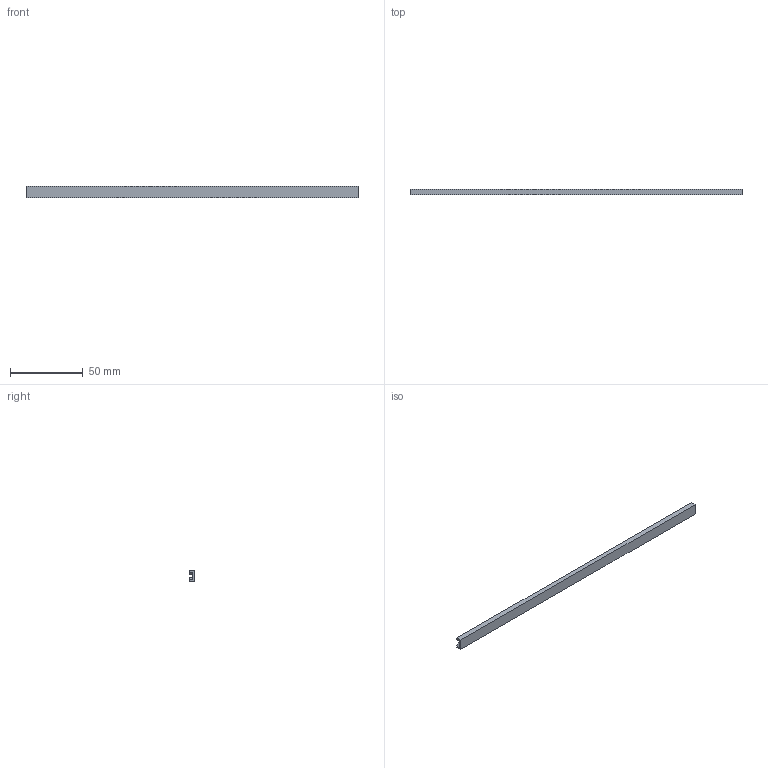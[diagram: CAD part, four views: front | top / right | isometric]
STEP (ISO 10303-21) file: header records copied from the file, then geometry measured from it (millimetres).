
FILE_DESCRIPTION (( 'STEP AP214' ), '1' );
FILE_NAME ('616-220-310.STEP', '2020-08-20T18:13:41', ( '' ), ( '' ), 'SwSTEP 2.0', 'SolidWorks 2020', '' );
FILE_SCHEMA (( 'AUTOMOTIVE_DESIGN' ));
Length unit declared in the file: inch
Products named in the file (1): 616-220-310
Bounding box: 228.6 x 3.71 x 7.92 mm (x, y, z)
Volume: 5534.2 mm3; surface area: 6360.8 mm2
Topology: 1 solids, 1 shells, 262 faces, 687 edges, 458 vertices
Faces by surface type: plane 168, bspline 94
Entity records: 13655 total; most frequent: CARTESIAN_POINT 7790, ORIENTED_EDGE 1374, DIRECTION 837, EDGE_CURVE 687, VECTOR 499, LINE 499, VERTEX_POINT 458, EDGE_LOOP 293
